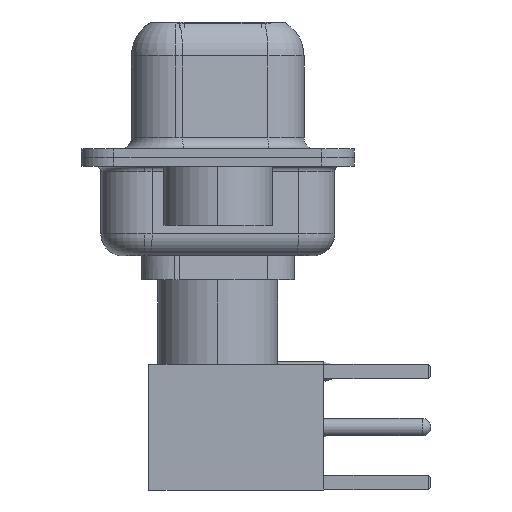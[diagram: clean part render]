
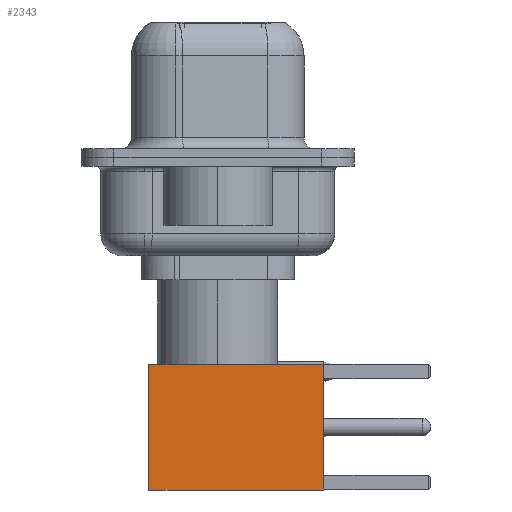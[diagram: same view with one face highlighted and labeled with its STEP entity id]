
A CAD part, left-side view. The second image highlights one B-rep face of the part: STEP entity #2343.
In plain terms, the highlighted face is planar.
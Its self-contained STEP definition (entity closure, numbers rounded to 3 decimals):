
#38 = CARTESIAN_POINT ( 'NONE',  ( -2.875, 2.875, 8. ) ) ;
#1759 = ORIENTED_EDGE ( 'NONE', *, *, #10169, .F. ) ;
#2343 = ADVANCED_FACE ( 'NONE', ( #8424 ), #23481, .T. ) ;
#2582 = CARTESIAN_POINT ( 'NONE',  ( 2.875, 2.875, 0. ) ) ;
#3671 = VECTOR ( 'NONE', #17084, 1000. ) ;
#4305 = VECTOR ( 'NONE', #21678, 1000. ) ;
#4368 = DIRECTION ( 'NONE',  ( 0., 0., 1. ) ) ;
#5795 = AXIS2_PLACEMENT_3D ( 'NONE', #19284, #25163, #4368 ) ;
#7500 = VERTEX_POINT ( 'NONE', #38 ) ;
#8276 = ORIENTED_EDGE ( 'NONE', *, *, #19290, .T. ) ;
#8424 = FACE_OUTER_BOUND ( 'NONE', #14461, .T. ) ;
#9140 = LINE ( 'NONE', #11653, #23247 ) ;
#10169 = EDGE_CURVE ( 'NONE', #7500, #20267, #9140, .T. ) ;
#10270 = CARTESIAN_POINT ( 'NONE',  ( 0., 2.875, 8. ) ) ;
#11653 = CARTESIAN_POINT ( 'NONE',  ( -2.875, 2.875, 0. ) ) ;
#11792 = ORIENTED_EDGE ( 'NONE', *, *, #23396, .T. ) ;
#12166 = CARTESIAN_POINT ( 'NONE',  ( 0., 2.875, 0. ) ) ;
#12764 = LINE ( 'NONE', #10270, #3671 ) ;
#13523 = VERTEX_POINT ( 'NONE', #18639 ) ;
#14461 = EDGE_LOOP ( 'NONE', ( #8276, #11792, #1759, #23021 ) ) ;
#16203 = LINE ( 'NONE', #12166, #16425 ) ;
#16425 = VECTOR ( 'NONE', #18724, 1000. ) ;
#17084 = DIRECTION ( 'NONE',  ( -1., 0., 0. ) ) ;
#18077 = CARTESIAN_POINT ( 'NONE',  ( -2.875, 2.875, 0. ) ) ;
#18639 = CARTESIAN_POINT ( 'NONE',  ( 2.875, 2.875, 8. ) ) ;
#18724 = DIRECTION ( 'NONE',  ( -1., 0., 0. ) ) ;
#19263 = VERTEX_POINT ( 'NONE', #2582 ) ;
#19284 = CARTESIAN_POINT ( 'NONE',  ( 2.875, 2.875, 0. ) ) ;
#19290 = EDGE_CURVE ( 'NONE', #13523, #19263, #23916, .T. ) ;
#19576 = CARTESIAN_POINT ( 'NONE',  ( 2.875, 2.875, 0. ) ) ;
#20267 = VERTEX_POINT ( 'NONE', #18077 ) ;
#21678 = DIRECTION ( 'NONE',  ( 0., 0., -1. ) ) ;
#22115 = DIRECTION ( 'NONE',  ( 0., 0., -1. ) ) ;
#23021 = ORIENTED_EDGE ( 'NONE', *, *, #26218, .F. ) ;
#23247 = VECTOR ( 'NONE', #22115, 1000. ) ;
#23396 = EDGE_CURVE ( 'NONE', #19263, #20267, #16203, .T. ) ;
#23481 = PLANE ( 'NONE',  #5795 ) ;
#23916 = LINE ( 'NONE', #19576, #4305 ) ;
#25163 = DIRECTION ( 'NONE',  ( 0., 1., 0. ) ) ;
#26218 = EDGE_CURVE ( 'NONE', #13523, #7500, #12764, .T. ) ;
